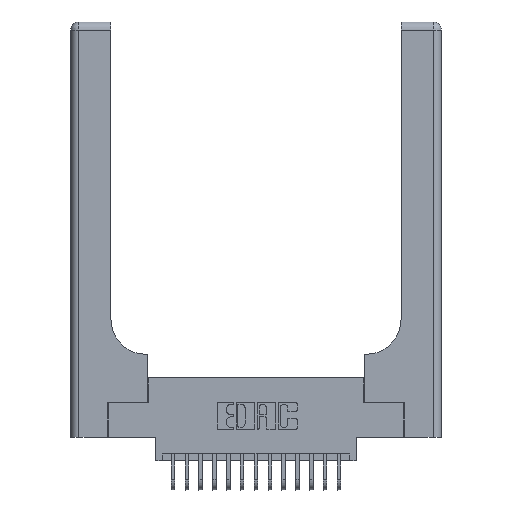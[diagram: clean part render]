
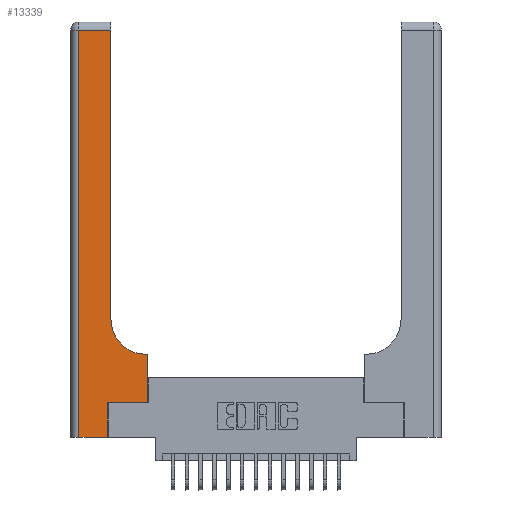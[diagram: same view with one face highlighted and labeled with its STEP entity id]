
A CAD part, top view. The second image highlights one B-rep face of the part: STEP entity #13339.
In plain terms, the highlighted planar face has unit normal (0, 0, 1).
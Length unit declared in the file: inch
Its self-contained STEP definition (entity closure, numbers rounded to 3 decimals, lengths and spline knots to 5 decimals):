
#260 = DIRECTION ( 'NONE',  ( -1., 0., 0. ) ) ;
#347 = PLANE ( 'NONE',  #10572 ) ;
#375 = LINE ( 'NONE', #13468, #21013 ) ;
#794 = EDGE_CURVE ( 'NONE', #16895, #4047, #5488, .T. ) ;
#841 = CARTESIAN_POINT ( 'NONE',  ( 0.5585, 0.25, 0.37 ) ) ;
#1339 = DIRECTION ( 'NONE',  ( 1., 0., 0. ) ) ;
#1451 = EDGE_CURVE ( 'NONE', #16400, #11370, #14943, .T. ) ;
#1459 = VECTOR ( 'NONE', #11529, 39.37008 ) ;
#2057 = ORIENTED_EDGE ( 'NONE', *, *, #794, .T. ) ;
#2141 = DIRECTION ( 'NONE',  ( 0., 0., -1. ) ) ;
#2579 = ORIENTED_EDGE ( 'NONE', *, *, #1451, .T. ) ;
#2742 = VERTEX_POINT ( 'NONE', #5101 ) ;
#2750 = CARTESIAN_POINT ( 'NONE',  ( 0.5415, 0.85, 0.37 ) ) ;
#3300 = DIRECTION ( 'NONE',  ( 0., 1., 0. ) ) ;
#3682 = DIRECTION ( 'NONE',  ( -1., 0., 0. ) ) ;
#4047 = VERTEX_POINT ( 'NONE', #16389 ) ;
#4450 = CARTESIAN_POINT ( 'NONE',  ( 0.5415, 0.6, 0.37 ) ) ;
#5101 = CARTESIAN_POINT ( 'NONE',  ( 0.06, 2.94, 0.37 ) ) ;
#5293 = CARTESIAN_POINT ( 'NONE',  ( 0.2915, 3., 0.37 ) ) ;
#5353 = EDGE_CURVE ( 'NONE', #4047, #12836, #19019, .T. ) ;
#5355 = ORIENTED_EDGE ( 'NONE', *, *, #7720, .T. ) ;
#5488 = CIRCLE ( 'NONE', #6761, 0.25 ) ;
#5489 = CARTESIAN_POINT ( 'NONE',  ( 0.5585, 0.6, 0.37 ) ) ;
#5687 = ORIENTED_EDGE ( 'NONE', *, *, #14981, .T. ) ;
#5702 = LINE ( 'NONE', #13626, #8573 ) ;
#6488 = DIRECTION ( 'NONE',  ( 0., -1., 0. ) ) ;
#6761 = AXIS2_PLACEMENT_3D ( 'NONE', #2750, #2141, #1339 ) ;
#7649 = VECTOR ( 'NONE', #3300, 39.37008 ) ;
#7720 = EDGE_CURVE ( 'NONE', #10952, #11701, #5702, .T. ) ;
#8310 = CARTESIAN_POINT ( 'NONE',  ( 0.269, 0.25, 0.37 ) ) ;
#8335 = CARTESIAN_POINT ( 'NONE',  ( 0., 2.94, 0.37 ) ) ;
#8502 = VECTOR ( 'NONE', #6488, 39.37008 ) ;
#8554 = VECTOR ( 'NONE', #11579, 39.37008 ) ;
#8573 = VECTOR ( 'NONE', #8811, 39.37008 ) ;
#8811 = DIRECTION ( 'NONE',  ( 1., 0., 0. ) ) ;
#8954 = EDGE_CURVE ( 'NONE', #19322, #16400, #12875, .T. ) ;
#9033 = LINE ( 'NONE', #20971, #8502 ) ;
#9775 = LINE ( 'NONE', #8335, #1459 ) ;
#9934 = FACE_OUTER_BOUND ( 'NONE', #17813, .T. ) ;
#10054 = EDGE_CURVE ( 'NONE', #12836, #2742, #9775, .T. ) ;
#10572 = AXIS2_PLACEMENT_3D ( 'NONE', #11915, #13544, #3682 ) ;
#10625 = VECTOR ( 'NONE', #19867, 39.37008 ) ;
#10931 = CARTESIAN_POINT ( 'NONE',  ( 0.06, 0., 0.37 ) ) ;
#10952 = VERTEX_POINT ( 'NONE', #10931 ) ;
#11370 = VERTEX_POINT ( 'NONE', #5489 ) ;
#11529 = DIRECTION ( 'NONE',  ( -1., 0., 0. ) ) ;
#11579 = DIRECTION ( 'NONE',  ( 1., 0., 0. ) ) ;
#11625 = CARTESIAN_POINT ( 'NONE',  ( 0.269, 0.25, 0.37 ) ) ;
#11701 = VERTEX_POINT ( 'NONE', #14437 ) ;
#11915 = CARTESIAN_POINT ( 'NONE',  ( 0., 3., 0.37 ) ) ;
#12836 = VERTEX_POINT ( 'NONE', #14101 ) ;
#12875 = LINE ( 'NONE', #8310, #8554 ) ;
#13339 = ADVANCED_FACE ( 'NONE', ( #9934 ), #347, .F. ) ;
#13468 = CARTESIAN_POINT ( 'NONE',  ( 0.2915, 0.6, 0.37 ) ) ;
#13544 = DIRECTION ( 'NONE',  ( 0., 0., -1. ) ) ;
#13626 = CARTESIAN_POINT ( 'NONE',  ( 0., 0., 0.37 ) ) ;
#14101 = CARTESIAN_POINT ( 'NONE',  ( 0.2915, 2.94, 0.37 ) ) ;
#14437 = CARTESIAN_POINT ( 'NONE',  ( 0.269, 0., 0.37 ) ) ;
#14943 = LINE ( 'NONE', #20137, #10625 ) ;
#14981 = EDGE_CURVE ( 'NONE', #2742, #10952, #9033, .T. ) ;
#16171 = EDGE_CURVE ( 'NONE', #11370, #16895, #375, .T. ) ;
#16389 = CARTESIAN_POINT ( 'NONE',  ( 0.2915, 0.85, 0.37 ) ) ;
#16400 = VERTEX_POINT ( 'NONE', #841 ) ;
#16714 = EDGE_CURVE ( 'NONE', #11701, #19322, #20512, .T. ) ;
#16895 = VERTEX_POINT ( 'NONE', #4450 ) ;
#17813 = EDGE_LOOP ( 'NONE', ( #18770, #19250, #5687, #5355, #19558, #19959, #2579, #20568, #2057 ) ) ;
#18530 = VECTOR ( 'NONE', #19904, 39.37008 ) ;
#18770 = ORIENTED_EDGE ( 'NONE', *, *, #5353, .T. ) ;
#19019 = LINE ( 'NONE', #5293, #18530 ) ;
#19250 = ORIENTED_EDGE ( 'NONE', *, *, #10054, .T. ) ;
#19322 = VERTEX_POINT ( 'NONE', #11625 ) ;
#19537 = CARTESIAN_POINT ( 'NONE',  ( 0.269, 0., 0.37 ) ) ;
#19558 = ORIENTED_EDGE ( 'NONE', *, *, #16714, .T. ) ;
#19867 = DIRECTION ( 'NONE',  ( 0., 1., 0. ) ) ;
#19904 = DIRECTION ( 'NONE',  ( 0., 1., 0. ) ) ;
#19959 = ORIENTED_EDGE ( 'NONE', *, *, #8954, .T. ) ;
#20137 = CARTESIAN_POINT ( 'NONE',  ( 0.5585, 0.25, 0.37 ) ) ;
#20512 = LINE ( 'NONE', #19537, #7649 ) ;
#20568 = ORIENTED_EDGE ( 'NONE', *, *, #16171, .T. ) ;
#20971 = CARTESIAN_POINT ( 'NONE',  ( 0.06, 3., 0.37 ) ) ;
#21013 = VECTOR ( 'NONE', #260, 39.37008 ) ;
